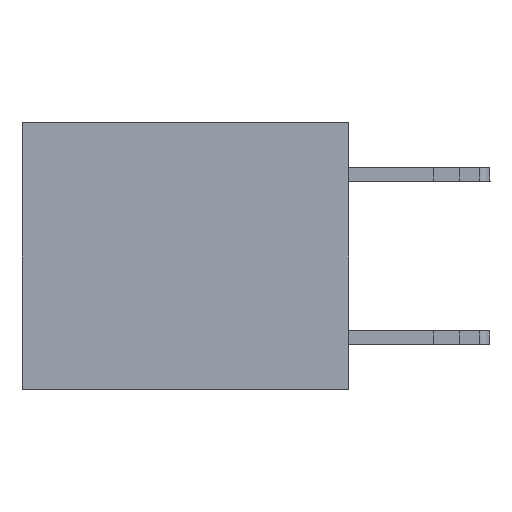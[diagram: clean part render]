
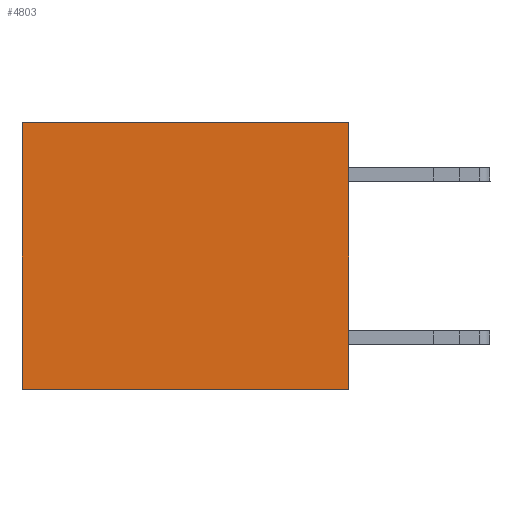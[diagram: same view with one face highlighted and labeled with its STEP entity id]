
A CAD part, left-side view. The second image highlights one B-rep face of the part: STEP entity #4803.
In plain terms, the highlighted planar face has unit normal (-1, 0, 0).
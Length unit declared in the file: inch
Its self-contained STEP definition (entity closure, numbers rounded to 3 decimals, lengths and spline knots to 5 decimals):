
#2102 = VECTOR ( 'NONE', #22367, 39.37008 ) ;
#3534 = EDGE_CURVE ( 'NONE', #6856, #5596, #10373, .T. ) ;
#4803 = ADVANCED_FACE ( 'NONE', ( #9462 ), #15192, .F. ) ;
#5307 = EDGE_CURVE ( 'NONE', #17190, #11089, #21740, .T. ) ;
#5596 = VERTEX_POINT ( 'NONE', #19585 ) ;
#6211 = CARTESIAN_POINT ( 'NONE',  ( 0.3165, 0., -0.49 ) ) ;
#6295 = DIRECTION ( 'NONE',  ( 1., 0., 0. ) ) ;
#6781 = CARTESIAN_POINT ( 'NONE',  ( 0.3165, 0.6, 0. ) ) ;
#6856 = VERTEX_POINT ( 'NONE', #18004 ) ;
#7384 = VECTOR ( 'NONE', #9421, 39.37008 ) ;
#8303 = CARTESIAN_POINT ( 'NONE',  ( 0.3165, 0., -0.49 ) ) ;
#8720 = ORIENTED_EDGE ( 'NONE', *, *, #5307, .T. ) ;
#9421 = DIRECTION ( 'NONE',  ( 0., 0., -1. ) ) ;
#9462 = FACE_OUTER_BOUND ( 'NONE', #12060, .T. ) ;
#9945 = DIRECTION ( 'NONE',  ( 0., 0., -1. ) ) ;
#10373 = LINE ( 'NONE', #8303, #17647 ) ;
#11089 = VERTEX_POINT ( 'NONE', #6781 ) ;
#11412 = CARTESIAN_POINT ( 'NONE',  ( 0.3165, 0., 0. ) ) ;
#12060 = EDGE_LOOP ( 'NONE', ( #12636, #19357, #22109, #8720 ) ) ;
#12344 = EDGE_CURVE ( 'NONE', #17190, #6856, #19374, .T. ) ;
#12636 = ORIENTED_EDGE ( 'NONE', *, *, #16504, .T. ) ;
#13018 = CARTESIAN_POINT ( 'NONE',  ( 0.3165, 0., 0. ) ) ;
#13248 = LINE ( 'NONE', #20057, #7384 ) ;
#14183 = VECTOR ( 'NONE', #22157, 39.37008 ) ;
#15192 = PLANE ( 'NONE',  #16654 ) ;
#15213 = CARTESIAN_POINT ( 'NONE',  ( 0.3165, 0., -0.49 ) ) ;
#16504 = EDGE_CURVE ( 'NONE', #11089, #5596, #13248, .T. ) ;
#16654 = AXIS2_PLACEMENT_3D ( 'NONE', #6211, #6295, #9945 ) ;
#17190 = VERTEX_POINT ( 'NONE', #13018 ) ;
#17647 = VECTOR ( 'NONE', #19073, 39.37008 ) ;
#18004 = CARTESIAN_POINT ( 'NONE',  ( 0.3165, 0., -0.49 ) ) ;
#19073 = DIRECTION ( 'NONE',  ( 0., 1., 0. ) ) ;
#19357 = ORIENTED_EDGE ( 'NONE', *, *, #3534, .F. ) ;
#19374 = LINE ( 'NONE', #15213, #2102 ) ;
#19585 = CARTESIAN_POINT ( 'NONE',  ( 0.3165, 0.6, -0.49 ) ) ;
#20057 = CARTESIAN_POINT ( 'NONE',  ( 0.3165, 0.6, -0.49 ) ) ;
#21740 = LINE ( 'NONE', #11412, #14183 ) ;
#22109 = ORIENTED_EDGE ( 'NONE', *, *, #12344, .F. ) ;
#22157 = DIRECTION ( 'NONE',  ( 0., 1., 0. ) ) ;
#22367 = DIRECTION ( 'NONE',  ( 0., 0., -1. ) ) ;
